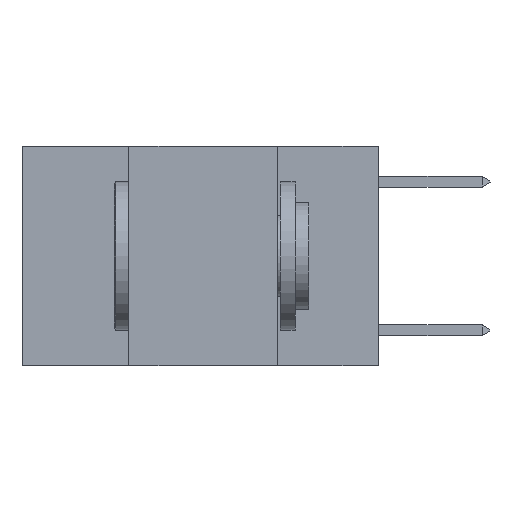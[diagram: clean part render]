
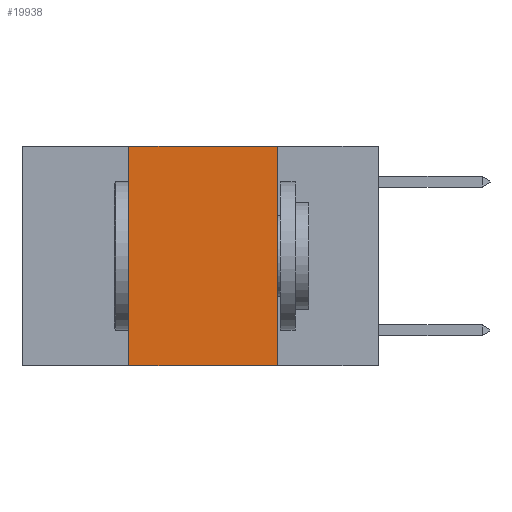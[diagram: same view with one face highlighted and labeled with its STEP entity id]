
A CAD part, left-side view. The second image highlights one B-rep face of the part: STEP entity #19938.
In plain terms, the highlighted planar face has unit normal (-1, 0, 0).
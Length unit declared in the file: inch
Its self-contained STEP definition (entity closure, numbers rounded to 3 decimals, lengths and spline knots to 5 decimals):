
#1666 = CARTESIAN_POINT ( 'NONE',  ( 0., 0.17, 0. ) ) ;
#2897 = VERTEX_POINT ( 'NONE', #16384 ) ;
#3176 = ORIENTED_EDGE ( 'NONE', *, *, #7142, .F. ) ;
#3873 = VECTOR ( 'NONE', #6293, 39.37008 ) ;
#4205 = CARTESIAN_POINT ( 'NONE',  ( 0., 0.6, -0.37 ) ) ;
#5741 = LINE ( 'NONE', #4205, #18682 ) ;
#5993 = CARTESIAN_POINT ( 'NONE',  ( 0., 0.42, 0. ) ) ;
#6293 = DIRECTION ( 'NONE',  ( 0., -1., 0. ) ) ;
#6499 = CARTESIAN_POINT ( 'NONE',  ( 0., 0.6, 0. ) ) ;
#6503 = CARTESIAN_POINT ( 'NONE',  ( 0., 0.17, 0. ) ) ;
#6756 = VERTEX_POINT ( 'NONE', #11923 ) ;
#7142 = EDGE_CURVE ( 'NONE', #2897, #11797, #9499, .T. ) ;
#7278 = LINE ( 'NONE', #1666, #11418 ) ;
#7575 = ORIENTED_EDGE ( 'NONE', *, *, #19166, .F. ) ;
#8003 = EDGE_CURVE ( 'NONE', #8909, #6756, #7278, .T. ) ;
#8226 = DIRECTION ( 'NONE',  ( 1., 0., 0. ) ) ;
#8367 = DIRECTION ( 'NONE',  ( 0., 0., -1. ) ) ;
#8909 = VERTEX_POINT ( 'NONE', #6503 ) ;
#9499 = LINE ( 'NONE', #18696, #18371 ) ;
#10041 = ORIENTED_EDGE ( 'NONE', *, *, #8003, .F. ) ;
#11418 = VECTOR ( 'NONE', #8367, 39.37008 ) ;
#11797 = VERTEX_POINT ( 'NONE', #5993 ) ;
#11923 = CARTESIAN_POINT ( 'NONE',  ( 0., 0.17, -0.37 ) ) ;
#13011 = EDGE_LOOP ( 'NONE', ( #10041, #7575, #3176, #13145 ) ) ;
#13145 = ORIENTED_EDGE ( 'NONE', *, *, #21364, .T. ) ;
#13205 = AXIS2_PLACEMENT_3D ( 'NONE', #6499, #8226, #20524 ) ;
#16292 = FACE_OUTER_BOUND ( 'NONE', #13011, .T. ) ;
#16384 = CARTESIAN_POINT ( 'NONE',  ( 0., 0.42, -0.37 ) ) ;
#17414 = LINE ( 'NONE', #20333, #3873 ) ;
#18306 = DIRECTION ( 'NONE',  ( 0., -1., 0. ) ) ;
#18371 = VECTOR ( 'NONE', #18899, 39.37008 ) ;
#18682 = VECTOR ( 'NONE', #18306, 39.37008 ) ;
#18696 = CARTESIAN_POINT ( 'NONE',  ( 0., 0.42, 0. ) ) ;
#18899 = DIRECTION ( 'NONE',  ( 0., 0., 1. ) ) ;
#19166 = EDGE_CURVE ( 'NONE', #11797, #8909, #17414, .T. ) ;
#19938 = ADVANCED_FACE ( 'NONE', ( #16292 ), #22145, .F. ) ;
#20333 = CARTESIAN_POINT ( 'NONE',  ( 0., 0.6, 0. ) ) ;
#20524 = DIRECTION ( 'NONE',  ( 0., 0., -1. ) ) ;
#21364 = EDGE_CURVE ( 'NONE', #2897, #6756, #5741, .T. ) ;
#22145 = PLANE ( 'NONE',  #13205 ) ;
